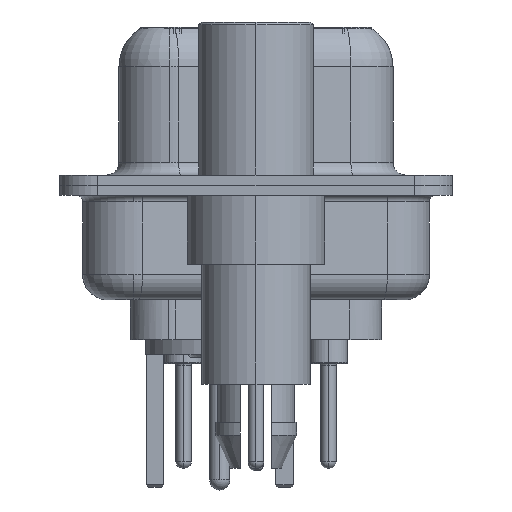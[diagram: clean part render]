
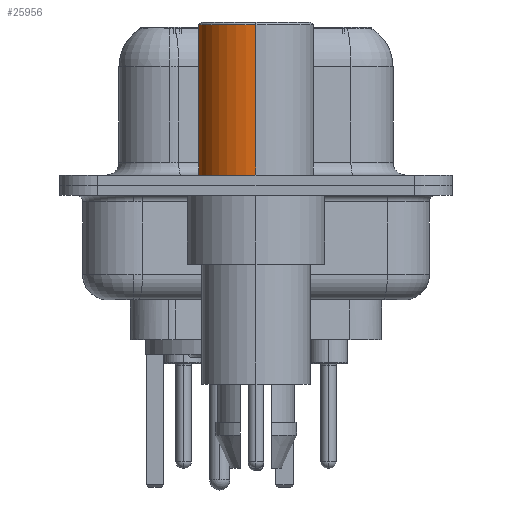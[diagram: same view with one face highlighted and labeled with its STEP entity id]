
A CAD part, left-side view. The second image highlights one B-rep face of the part: STEP entity #25956.
In plain terms, the highlighted cylindrical face has radius 2.25 mm (diameter 4.5 mm), a partial arc.
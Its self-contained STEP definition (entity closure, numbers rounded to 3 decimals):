
#429 = DIRECTION ( 'NONE',  ( 1., 0., 0. ) ) ;
#501 = CARTESIAN_POINT ( 'NONE',  ( -2.25, 0., 0.4 ) ) ;
#1071 = DIRECTION ( 'NONE',  ( 0., 0., 1. ) ) ;
#1607 = FACE_OUTER_BOUND ( 'NONE', #8336, .T. ) ;
#1999 = ORIENTED_EDGE ( 'NONE', *, *, #3581, .T. ) ;
#2989 = VECTOR ( 'NONE', #24389, 1000. ) ;
#3581 = EDGE_CURVE ( 'NONE', #23124, #22855, #31174, .T. ) ;
#3623 = CARTESIAN_POINT ( 'NONE',  ( 0., 0., 0.4 ) ) ;
#4873 = VERTEX_POINT ( 'NONE', #33456 ) ;
#5748 = DIRECTION ( 'NONE',  ( 0., 0., 1. ) ) ;
#8336 = EDGE_LOOP ( 'NONE', ( #1999, #30632, #34174, #26708 ) ) ;
#10777 = EDGE_CURVE ( 'NONE', #4873, #23612, #26511, .T. ) ;
#11659 = LINE ( 'NONE', #32121, #2989 ) ;
#12100 = CARTESIAN_POINT ( 'NONE',  ( 0., 0., 0.581 ) ) ;
#12193 = AXIS2_PLACEMENT_3D ( 'NONE', #19423, #5748, #429 ) ;
#15082 = CARTESIAN_POINT ( 'NONE',  ( 2.25, 0., 0.581 ) ) ;
#15479 = CARTESIAN_POINT ( 'NONE',  ( 2.25, 0., 0.4 ) ) ;
#18000 = LINE ( 'NONE', #15082, #25355 ) ;
#19423 = CARTESIAN_POINT ( 'NONE',  ( 0., 0., 6.3 ) ) ;
#19858 = EDGE_CURVE ( 'NONE', #22855, #23612, #11659, .T. ) ;
#20290 = AXIS2_PLACEMENT_3D ( 'NONE', #12100, #1071, #28437 ) ;
#20394 = DIRECTION ( 'NONE',  ( 0., 0., 1. ) ) ;
#20673 = CYLINDRICAL_SURFACE ( 'NONE', #20290, 2.25 ) ;
#22855 = VERTEX_POINT ( 'NONE', #501 ) ;
#23124 = VERTEX_POINT ( 'NONE', #15479 ) ;
#23612 = VERTEX_POINT ( 'NONE', #25550 ) ;
#24389 = DIRECTION ( 'NONE',  ( 0., 0., 1. ) ) ;
#25280 = DIRECTION ( 'NONE',  ( 0., 0., 1. ) ) ;
#25355 = VECTOR ( 'NONE', #20394, 1000. ) ;
#25550 = CARTESIAN_POINT ( 'NONE',  ( -2.25, 0., 6.3 ) ) ;
#25956 = ADVANCED_FACE ( 'NONE', ( #1607 ), #20673, .T. ) ;
#26511 = CIRCLE ( 'NONE', #12193, 2.25 ) ;
#26708 = ORIENTED_EDGE ( 'NONE', *, *, #26947, .F. ) ;
#26947 = EDGE_CURVE ( 'NONE', #23124, #4873, #18000, .T. ) ;
#28437 = DIRECTION ( 'NONE',  ( 1., 0., 0. ) ) ;
#30188 = AXIS2_PLACEMENT_3D ( 'NONE', #3623, #25280, #31198 ) ;
#30632 = ORIENTED_EDGE ( 'NONE', *, *, #19858, .T. ) ;
#31174 = CIRCLE ( 'NONE', #30188, 2.25 ) ;
#31198 = DIRECTION ( 'NONE',  ( 1., 0., 0. ) ) ;
#32121 = CARTESIAN_POINT ( 'NONE',  ( -2.25, 0., 0.581 ) ) ;
#33456 = CARTESIAN_POINT ( 'NONE',  ( 2.25, 0., 6.3 ) ) ;
#34174 = ORIENTED_EDGE ( 'NONE', *, *, #10777, .F. ) ;
